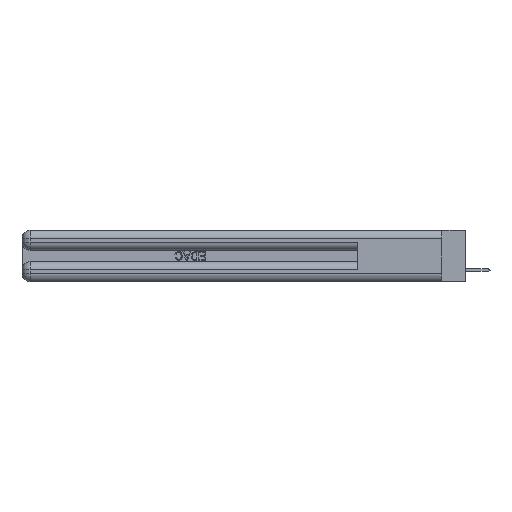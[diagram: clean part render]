
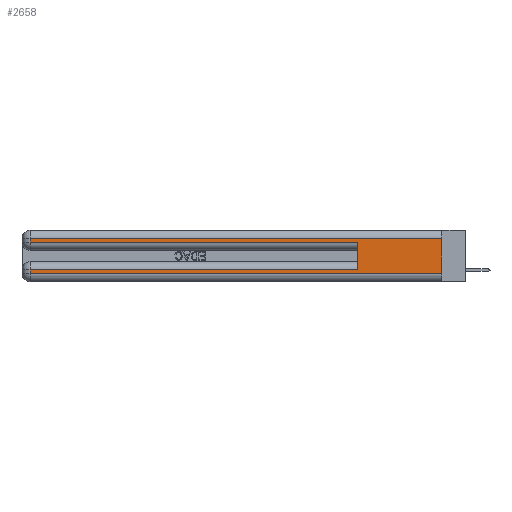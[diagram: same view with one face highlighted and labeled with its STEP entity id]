
A CAD part, left-side view. The second image highlights one B-rep face of the part: STEP entity #2658.
In plain terms, the highlighted planar face has unit normal (-1, 0, 0).
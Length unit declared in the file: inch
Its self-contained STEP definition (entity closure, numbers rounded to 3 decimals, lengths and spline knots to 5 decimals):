
#1202 = EDGE_CURVE ( 'NONE', #42510, #34085, #23484, .T. ) ;
#1908 = LINE ( 'NONE', #39945, #39667 ) ;
#2234 = VECTOR ( 'NONE', #26819, 39.37008 ) ;
#2658 = ADVANCED_FACE ( 'NONE', ( #13524 ), #34837, .F. ) ;
#4990 = DIRECTION ( 'NONE',  ( 1., 0., 0. ) ) ;
#5175 = CARTESIAN_POINT ( 'NONE',  ( 0., 0.6, 0.085 ) ) ;
#6270 = LINE ( 'NONE', #13175, #36303 ) ;
#7616 = CARTESIAN_POINT ( 'NONE',  ( 0., 0., 0.06 ) ) ;
#7670 = DIRECTION ( 'NONE',  ( 0., 0., -1. ) ) ;
#8624 = ORIENTED_EDGE ( 'NONE', *, *, #10811, .T. ) ;
#9177 = DIRECTION ( 'NONE',  ( 0., 0., -1. ) ) ;
#9342 = CARTESIAN_POINT ( 'NONE',  ( 0., 0., 0.31 ) ) ;
#9839 = EDGE_LOOP ( 'NONE', ( #38915, #11360, #8624, #20224, #29675, #28609, #16965, #15786 ) ) ;
#10150 = EDGE_CURVE ( 'NONE', #42510, #22225, #6270, .T. ) ;
#10470 = DIRECTION ( 'NONE',  ( 0., 0., 1. ) ) ;
#10811 = EDGE_CURVE ( 'NONE', #22225, #12296, #16602, .T. ) ;
#10912 = CARTESIAN_POINT ( 'NONE',  ( 0., 2.94, 0.06 ) ) ;
#11191 = CARTESIAN_POINT ( 'NONE',  ( 0., 2.94, 0.285 ) ) ;
#11360 = ORIENTED_EDGE ( 'NONE', *, *, #10150, .T. ) ;
#12296 = VERTEX_POINT ( 'NONE', #11191 ) ;
#13175 = CARTESIAN_POINT ( 'NONE',  ( 0., 0., 0.31 ) ) ;
#13524 = FACE_OUTER_BOUND ( 'NONE', #9839, .T. ) ;
#14611 = LINE ( 'NONE', #30288, #2234 ) ;
#15786 = ORIENTED_EDGE ( 'NONE', *, *, #39800, .T. ) ;
#16602 = LINE ( 'NONE', #16838, #17851 ) ;
#16838 = CARTESIAN_POINT ( 'NONE',  ( 0., 2.94, 0.37 ) ) ;
#16965 = ORIENTED_EDGE ( 'NONE', *, *, #21627, .T. ) ;
#17081 = VERTEX_POINT ( 'NONE', #26557 ) ;
#17851 = VECTOR ( 'NONE', #43441, 39.37008 ) ;
#18241 = CARTESIAN_POINT ( 'NONE',  ( 0., 0., 0.37 ) ) ;
#20224 = ORIENTED_EDGE ( 'NONE', *, *, #41294, .T. ) ;
#20591 = VECTOR ( 'NONE', #7670, 39.37008 ) ;
#21627 = EDGE_CURVE ( 'NONE', #17081, #50570, #24541, .T. ) ;
#22225 = VERTEX_POINT ( 'NONE', #26461 ) ;
#23258 = VERTEX_POINT ( 'NONE', #35293 ) ;
#23484 = LINE ( 'NONE', #44897, #34514 ) ;
#24541 = LINE ( 'NONE', #28044, #20591 ) ;
#24556 = DIRECTION ( 'NONE',  ( 0., 0., -1. ) ) ;
#24759 = EDGE_CURVE ( 'NONE', #27113, #17081, #14611, .T. ) ;
#26461 = CARTESIAN_POINT ( 'NONE',  ( 0., 2.94, 0.31 ) ) ;
#26557 = CARTESIAN_POINT ( 'NONE',  ( 0., 2.94, 0.085 ) ) ;
#26819 = DIRECTION ( 'NONE',  ( 0., 1., 0. ) ) ;
#27113 = VERTEX_POINT ( 'NONE', #5175 ) ;
#28044 = CARTESIAN_POINT ( 'NONE',  ( 0., 2.94, 0.37 ) ) ;
#28609 = ORIENTED_EDGE ( 'NONE', *, *, #24759, .T. ) ;
#29675 = ORIENTED_EDGE ( 'NONE', *, *, #44064, .F. ) ;
#30288 = CARTESIAN_POINT ( 'NONE',  ( 0., 0., 0.085 ) ) ;
#34085 = VERTEX_POINT ( 'NONE', #7616 ) ;
#34101 = DIRECTION ( 'NONE',  ( 0., 1., 0. ) ) ;
#34514 = VECTOR ( 'NONE', #24556, 39.37008 ) ;
#34837 = PLANE ( 'NONE',  #40258 ) ;
#35293 = CARTESIAN_POINT ( 'NONE',  ( 0., 0.6, 0.285 ) ) ;
#36303 = VECTOR ( 'NONE', #34101, 39.37008 ) ;
#38915 = ORIENTED_EDGE ( 'NONE', *, *, #1202, .F. ) ;
#39667 = VECTOR ( 'NONE', #10470, 39.37008 ) ;
#39800 = EDGE_CURVE ( 'NONE', #50570, #34085, #49206, .T. ) ;
#39945 = CARTESIAN_POINT ( 'NONE',  ( 0., 0.6, 0.145 ) ) ;
#40258 = AXIS2_PLACEMENT_3D ( 'NONE', #18241, #4990, #9177 ) ;
#41031 = DIRECTION ( 'NONE',  ( 0., -1., 0. ) ) ;
#41170 = DIRECTION ( 'NONE',  ( 0., -1., 0. ) ) ;
#41294 = EDGE_CURVE ( 'NONE', #12296, #23258, #42593, .T. ) ;
#42510 = VERTEX_POINT ( 'NONE', #9342 ) ;
#42593 = LINE ( 'NONE', #49794, #46493 ) ;
#43441 = DIRECTION ( 'NONE',  ( 0., 0., -1. ) ) ;
#44064 = EDGE_CURVE ( 'NONE', #27113, #23258, #1908, .T. ) ;
#44897 = CARTESIAN_POINT ( 'NONE',  ( 0., 0., 0.37 ) ) ;
#46493 = VECTOR ( 'NONE', #41170, 39.37008 ) ;
#49206 = LINE ( 'NONE', #49672, #49840 ) ;
#49672 = CARTESIAN_POINT ( 'NONE',  ( 0., 0., 0.06 ) ) ;
#49794 = CARTESIAN_POINT ( 'NONE',  ( 0., 0., 0.285 ) ) ;
#49840 = VECTOR ( 'NONE', #41031, 39.37008 ) ;
#50570 = VERTEX_POINT ( 'NONE', #10912 ) ;
